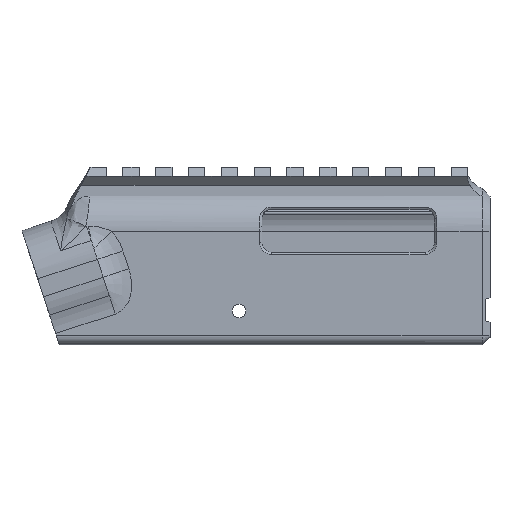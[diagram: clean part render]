
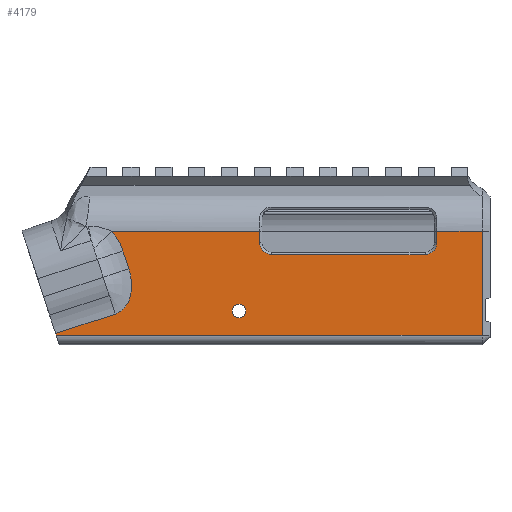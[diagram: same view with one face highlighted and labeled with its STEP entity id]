
A CAD part, left-side view. The second image highlights one B-rep face of the part: STEP entity #4179.
In plain terms, the highlighted planar face has unit normal (-1, 0, 0).
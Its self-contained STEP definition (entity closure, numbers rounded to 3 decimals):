
#28=FACE_BOUND('',#605,.T.);
#166=PLANE('',#4475);
#374=FACE_OUTER_BOUND('',#604,.T.);
#604=EDGE_LOOP('',(#3553,#3554,#3555,#3556,#3557,#3558,#3559,#3560,#3561,
#3562,#3563,#3564,#3565,#3566));
#605=EDGE_LOOP('',(#3567));
#764=CIRCLE('',#4476,3.75);
#765=CIRCLE('',#4477,3.75);
#766=CIRCLE('',#4478,2.175);
#993=LINE('',#6685,#1427);
#995=LINE('',#6714,#1429);
#1118=LINE('',#7435,#1552);
#1119=LINE('',#7589,#1553);
#1120=LINE('',#7591,#1554);
#1121=LINE('',#7593,#1555);
#1122=LINE('',#7594,#1556);
#1123=LINE('',#7596,#1557);
#1124=LINE('',#7600,#1558);
#1125=LINE('',#7603,#1559);
#1427=VECTOR('',#5000,10.);
#1429=VECTOR('',#5006,10.);
#1552=VECTOR('',#5289,16.161);
#1553=VECTOR('',#5304,10.);
#1554=VECTOR('',#5305,10.);
#1555=VECTOR('',#5306,10.);
#1556=VECTOR('',#5307,10.);
#1557=VECTOR('',#5308,10.);
#1558=VECTOR('',#5311,10.);
#1559=VECTOR('',#5314,10.);
#1733=B_SPLINE_CURVE_WITH_KNOTS('',3,(#7455,#7456,#7457,#7458),
 .UNSPECIFIED.,.F.,.F.,(4,4),(-6.622,-5.894),
 .UNSPECIFIED.);
#1734=B_SPLINE_CURVE_WITH_KNOTS('',3,(#7518,#7519,#7520,#7521,#7522,#7523,
#7524,#7525,#7526,#7527,#7528,#7529,#7530,#7531),.UNSPECIFIED.,.F.,.F.,
(4,1,1,1,1,1,1,1,1,1,1,4),(-8.277,-8.041,-7.804,
-7.568,-7.39,-7.095,-6.977,
-6.858,-6.74,-6.681,-6.652,
-6.622),.UNSPECIFIED.);
#1933=VERTEX_POINT('',#6677);
#1934=VERTEX_POINT('',#6684);
#1940=VERTEX_POINT('',#6711);
#1941=VERTEX_POINT('',#6713);
#2009=VERTEX_POINT('',#7428);
#2012=VERTEX_POINT('',#7433);
#2014=VERTEX_POINT('',#7515);
#2016=VERTEX_POINT('',#7588);
#2017=VERTEX_POINT('',#7590);
#2018=VERTEX_POINT('',#7592);
#2019=VERTEX_POINT('',#7595);
#2020=VERTEX_POINT('',#7597);
#2021=VERTEX_POINT('',#7599);
#2022=VERTEX_POINT('',#7601);
#2023=VERTEX_POINT('',#7604);
#2384=EDGE_CURVE('',#1934,#1933,#993,.T.);
#2391=EDGE_CURVE('',#1941,#1940,#995,.T.);
#2542=EDGE_CURVE('',#2012,#2009,#1118,.T.);
#2545=EDGE_CURVE('',#2009,#1933,#1733,.T.);
#2547=EDGE_CURVE('',#2014,#2012,#1734,.T.);
#2551=EDGE_CURVE('',#2016,#2014,#1119,.T.);
#2552=EDGE_CURVE('',#2016,#2017,#1120,.T.);
#2553=EDGE_CURVE('',#2018,#2017,#1121,.T.);
#2554=EDGE_CURVE('',#1941,#2018,#1122,.T.);
#2555=EDGE_CURVE('',#2019,#1940,#1123,.T.);
#2556=EDGE_CURVE('',#2020,#2019,#764,.T.);
#2557=EDGE_CURVE('',#2021,#2020,#1124,.T.);
#2558=EDGE_CURVE('',#2022,#2021,#765,.T.);
#2559=EDGE_CURVE('',#1934,#2022,#1125,.T.);
#2560=EDGE_CURVE('',#2023,#2023,#766,.T.);
#3553=ORIENTED_EDGE('',*,*,#2545,.F.);
#3554=ORIENTED_EDGE('',*,*,#2542,.F.);
#3555=ORIENTED_EDGE('',*,*,#2547,.F.);
#3556=ORIENTED_EDGE('',*,*,#2551,.F.);
#3557=ORIENTED_EDGE('',*,*,#2552,.T.);
#3558=ORIENTED_EDGE('',*,*,#2553,.F.);
#3559=ORIENTED_EDGE('',*,*,#2554,.F.);
#3560=ORIENTED_EDGE('',*,*,#2391,.T.);
#3561=ORIENTED_EDGE('',*,*,#2555,.F.);
#3562=ORIENTED_EDGE('',*,*,#2556,.F.);
#3563=ORIENTED_EDGE('',*,*,#2557,.F.);
#3564=ORIENTED_EDGE('',*,*,#2558,.F.);
#3565=ORIENTED_EDGE('',*,*,#2559,.F.);
#3566=ORIENTED_EDGE('',*,*,#2384,.T.);
#3567=ORIENTED_EDGE('',*,*,#2560,.T.);
#4179=ADVANCED_FACE('',(#374,#28),#166,.T.);
#4475=AXIS2_PLACEMENT_3D('',#7587,#5302,#5303);
#4476=AXIS2_PLACEMENT_3D('',#7598,#5309,#5310);
#4477=AXIS2_PLACEMENT_3D('',#7602,#5312,#5313);
#4478=AXIS2_PLACEMENT_3D('',#7605,#5315,#5316);
#5000=DIRECTION('',(0.,1.,0.));
#5006=DIRECTION('',(0.,1.,0.));
#5289=DIRECTION('',(0.,0.311,0.95));
#5302=DIRECTION('center_axis',(-1.,0.,0.));
#5303=DIRECTION('ref_axis',(0.,0.,1.));
#5304=DIRECTION('',(0.,-0.95,0.311));
#5305=DIRECTION('',(0.,-0.311,-0.95));
#5306=DIRECTION('',(0.,1.,0.));
#5307=DIRECTION('',(0.,0.,-1.));
#5308=DIRECTION('',(0.,0.,1.));
#5309=DIRECTION('center_axis',(-1.,0.,0.));
#5310=DIRECTION('ref_axis',(0.,-0.707,-0.707));
#5311=DIRECTION('',(0.,-1.,0.));
#5312=DIRECTION('center_axis',(-1.,0.,0.));
#5313=DIRECTION('ref_axis',(0.,0.707,-0.707));
#5314=DIRECTION('',(0.,0.,-1.));
#5315=DIRECTION('center_axis',(1.,0.,0.));
#5316=DIRECTION('ref_axis',(0.,-1.,0.));
#6677=CARTESIAN_POINT('',(-13.7,120.647,36.2));
#6684=CARTESIAN_POINT('',(-13.7,73.45,36.2));
#6685=CARTESIAN_POINT('',(-13.7,0.,36.2));
#6711=CARTESIAN_POINT('',(-13.7,16.95,36.2));
#6713=CARTESIAN_POINT('',(-13.7,2.5,36.2));
#6714=CARTESIAN_POINT('',(-13.7,0.,36.2));
#7428=CARTESIAN_POINT('',(-13.7,117.022,29.935));
#7433=CARTESIAN_POINT('',(-13.7,115.16,24.254));
#7435=CARTESIAN_POINT('',(-13.7,115.16,24.254));
#7455=CARTESIAN_POINT('Ctrl Pts',(-13.7,117.022,29.935));
#7456=CARTESIAN_POINT('Ctrl Pts',(-13.7,117.777,32.242));
#7457=CARTESIAN_POINT('Ctrl Pts',(-13.7,118.965,34.427));
#7458=CARTESIAN_POINT('Ctrl Pts',(-13.7,120.647,36.2));
#7515=CARTESIAN_POINT('',(-13.7,119.455,9.829));
#7518=CARTESIAN_POINT('Ctrl Pts',(-13.7,119.455,9.829));
#7519=CARTESIAN_POINT('Ctrl Pts',(-13.7,118.703,10.075));
#7520=CARTESIAN_POINT('Ctrl Pts',(-13.7,117.293,10.868));
#7521=CARTESIAN_POINT('Ctrl Pts',(-13.7,115.734,12.709));
#7522=CARTESIAN_POINT('Ctrl Pts',(-13.7,114.84,14.709));
#7523=CARTESIAN_POINT('Ctrl Pts',(-13.7,114.301,17.044));
#7524=CARTESIAN_POINT('Ctrl Pts',(-13.7,114.221,19.02));
#7525=CARTESIAN_POINT('Ctrl Pts',(-13.7,114.372,20.796));
#7526=CARTESIAN_POINT('Ctrl Pts',(-13.7,114.556,21.964));
#7527=CARTESIAN_POINT('Ctrl Pts',(-13.7,114.772,22.929));
#7528=CARTESIAN_POINT('Ctrl Pts',(-13.7,114.956,23.595));
#7529=CARTESIAN_POINT('Ctrl Pts',(-13.7,115.07,23.973));
#7530=CARTESIAN_POINT('Ctrl Pts',(-13.7,115.13,24.161));
#7531=CARTESIAN_POINT('Ctrl Pts',(-13.7,115.16,24.254));
#7587=CARTESIAN_POINT('Origin',(-13.7,0.,0.));
#7588=CARTESIAN_POINT('',(-13.7,138.461,3.602));
#7589=CARTESIAN_POINT('',(-13.7,138.461,3.602));
#7590=CARTESIAN_POINT('',(-13.7,138.264,3.));
#7591=CARTESIAN_POINT('',(-13.7,130.627,-20.31));
#7592=CARTESIAN_POINT('',(-13.7,2.5,3.));
#7593=CARTESIAN_POINT('',(-13.7,0.,3.));
#7594=CARTESIAN_POINT('',(-13.7,2.5,12.475));
#7595=CARTESIAN_POINT('',(-13.7,16.95,32.55));
#7596=CARTESIAN_POINT('',(-13.7,16.95,21.65));
#7597=CARTESIAN_POINT('',(-13.7,20.7,28.8));
#7598=CARTESIAN_POINT('Origin',(-13.7,20.7,32.55));
#7599=CARTESIAN_POINT('',(-13.7,69.7,28.8));
#7600=CARTESIAN_POINT('',(-13.7,8.85,28.8));
#7601=CARTESIAN_POINT('',(-13.7,73.45,32.55));
#7602=CARTESIAN_POINT('Origin',(-13.7,69.7,32.55));
#7603=CARTESIAN_POINT('',(-13.7,73.45,14.775));
#7604=CARTESIAN_POINT('',(-13.7,82.2,10.775));
#7605=CARTESIAN_POINT('Origin',(-13.7,80.025,10.775));
